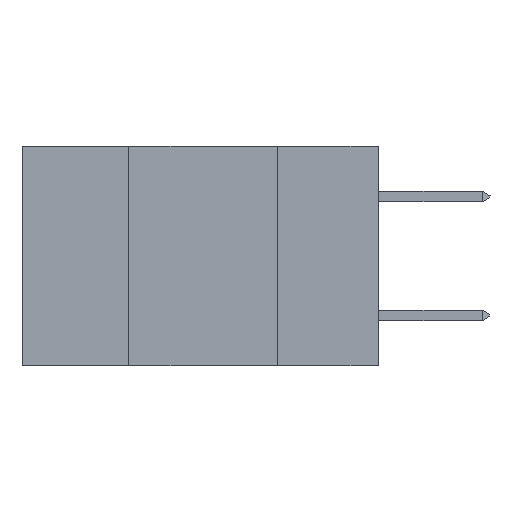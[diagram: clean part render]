
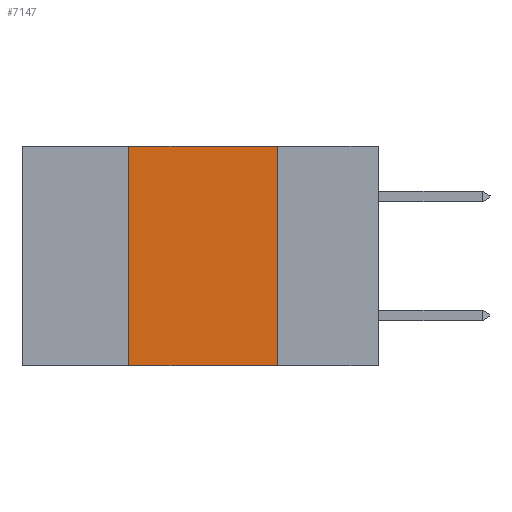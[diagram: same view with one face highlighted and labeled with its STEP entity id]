
A CAD part, left-side view. The second image highlights one B-rep face of the part: STEP entity #7147.
In plain terms, the highlighted planar face has unit normal (-1, 0, 0).
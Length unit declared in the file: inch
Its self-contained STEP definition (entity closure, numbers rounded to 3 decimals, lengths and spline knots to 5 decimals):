
#67 = VECTOR ( 'NONE', #9761, 39.37008 ) ;
#904 = CARTESIAN_POINT ( 'NONE',  ( 0., 0.6, 0. ) ) ;
#959 = EDGE_CURVE ( 'NONE', #8405, #9850, #6399, .T. ) ;
#990 = ORIENTED_EDGE ( 'NONE', *, *, #959, .F. ) ;
#1026 = VECTOR ( 'NONE', #3493, 39.37008 ) ;
#1400 = CARTESIAN_POINT ( 'NONE',  ( 0., 0.17, 0. ) ) ;
#1598 = DIRECTION ( 'NONE',  ( 0., -1., 0. ) ) ;
#1758 = FACE_OUTER_BOUND ( 'NONE', #3855, .T. ) ;
#2571 = CARTESIAN_POINT ( 'NONE',  ( 0., 0.6, 0. ) ) ;
#2710 = CARTESIAN_POINT ( 'NONE',  ( 0., 0.17, -0.37 ) ) ;
#2714 = LINE ( 'NONE', #904, #1026 ) ;
#3360 = CARTESIAN_POINT ( 'NONE',  ( 0., 0.6, -0.37 ) ) ;
#3493 = DIRECTION ( 'NONE',  ( 0., -1., 0. ) ) ;
#3855 = EDGE_LOOP ( 'NONE', ( #6713, #10851, #990, #6457 ) ) ;
#5149 = VECTOR ( 'NONE', #1598, 39.37008 ) ;
#6399 = LINE ( 'NONE', #6459, #67 ) ;
#6457 = ORIENTED_EDGE ( 'NONE', *, *, #8835, .T. ) ;
#6459 = CARTESIAN_POINT ( 'NONE',  ( 0., 0.42, -0.37 ) ) ;
#6706 = DIRECTION ( 'NONE',  ( 1., 0., 0. ) ) ;
#6713 = ORIENTED_EDGE ( 'NONE', *, *, #7473, .F. ) ;
#7034 = CARTESIAN_POINT ( 'NONE',  ( 0., 0.42, 0. ) ) ;
#7147 = ADVANCED_FACE ( 'NONE', ( #1758 ), #7647, .F. ) ;
#7244 = CARTESIAN_POINT ( 'NONE',  ( 0., 0.17, -0.37 ) ) ;
#7473 = EDGE_CURVE ( 'NONE', #10927, #10759, #9959, .T. ) ;
#7539 = CARTESIAN_POINT ( 'NONE',  ( 0., 0.42, -0.37 ) ) ;
#7647 = PLANE ( 'NONE',  #10442 ) ;
#8136 = DIRECTION ( 'NONE',  ( 0., 0., -1. ) ) ;
#8405 = VERTEX_POINT ( 'NONE', #7539 ) ;
#8649 = VECTOR ( 'NONE', #8136, 39.37008 ) ;
#8835 = EDGE_CURVE ( 'NONE', #8405, #10759, #9240, .T. ) ;
#9240 = LINE ( 'NONE', #3360, #5149 ) ;
#9344 = DIRECTION ( 'NONE',  ( 0., 0., -1. ) ) ;
#9489 = EDGE_CURVE ( 'NONE', #9850, #10927, #2714, .T. ) ;
#9761 = DIRECTION ( 'NONE',  ( 0., 0., 1. ) ) ;
#9850 = VERTEX_POINT ( 'NONE', #7034 ) ;
#9959 = LINE ( 'NONE', #7244, #8649 ) ;
#10442 = AXIS2_PLACEMENT_3D ( 'NONE', #2571, #6706, #9344 ) ;
#10759 = VERTEX_POINT ( 'NONE', #2710 ) ;
#10851 = ORIENTED_EDGE ( 'NONE', *, *, #9489, .F. ) ;
#10927 = VERTEX_POINT ( 'NONE', #1400 ) ;
